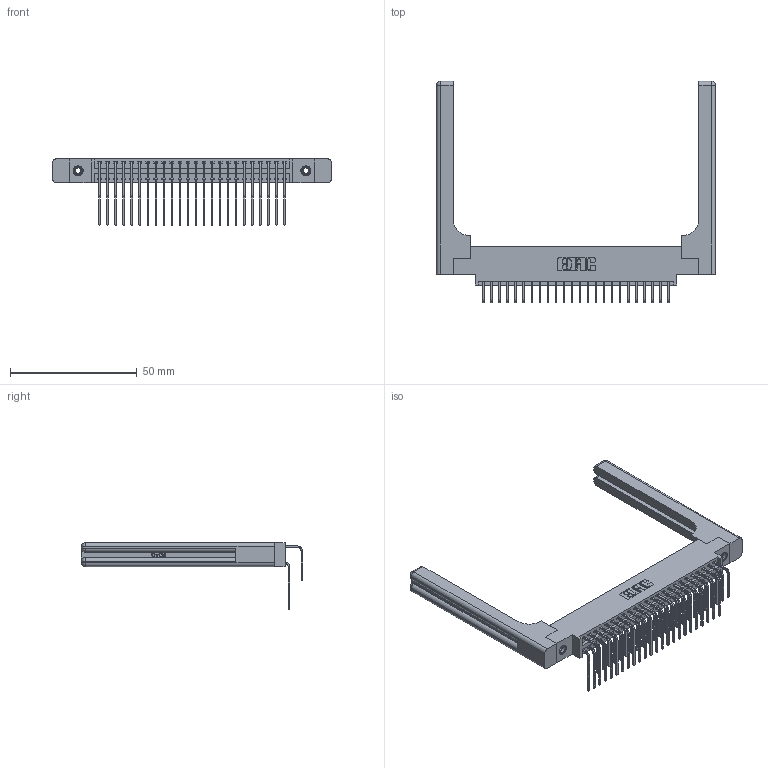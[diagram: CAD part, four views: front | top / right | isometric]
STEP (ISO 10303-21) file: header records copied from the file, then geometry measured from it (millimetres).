
FILE_DESCRIPTION (( 'STEP AP203' ), '1' );
FILE_NAME ('396-048-558-858.STEP', '2019-11-03T08:21:51', ( '' ), ( '' ), 'SwSTEP 2.0', 'SolidWorks 2016', '' );
FILE_SCHEMA (( 'CONFIG_CONTROL_DESIGN' ));
Length unit declared in the file: inch
Products named in the file (6): 345-292-001_558 559 Tail - 1; 345-250-001_345-250-001-102; 345-292-001_558 Tail - 2; 346-220-058_345-220-058; 346 Part_0.170 Offset - 0.156 Dia-TH; 396-048-558-858
Assembly tree (53 placements, depth 2):
  396-048-558-858
    346 Part_0.170 Offset - 0.156 Dia-TH
    345-292-001_558 559 Tail - 1  x24
    345-292-001_558 Tail - 2  x24
    345-250-001_345-250-001-102  x2
    346-220-058_345-220-058  x2
Bounding box: 110.26 x 87.44 x 26.16 mm (x, y, z)
Volume: 18228.6 mm3; surface area: 20952.9 mm2
Topology: 53 solids, 53 shells, 2974 faces, 8735 edges, 5738 vertices
Faces by surface type: plane 2004, cylinder 910, bspline 36, cone 12, sphere 8, torus 4
Entity records: 25184 total; most frequent: CARTESIAN_POINT 5236, ORIENTED_EDGE 3916, DIRECTION 3570, EDGE_CURVE 1958, LINE 1598, VECTOR 1598, VERTEX_POINT 1294, AXIS2_PLACEMENT_3D 986
